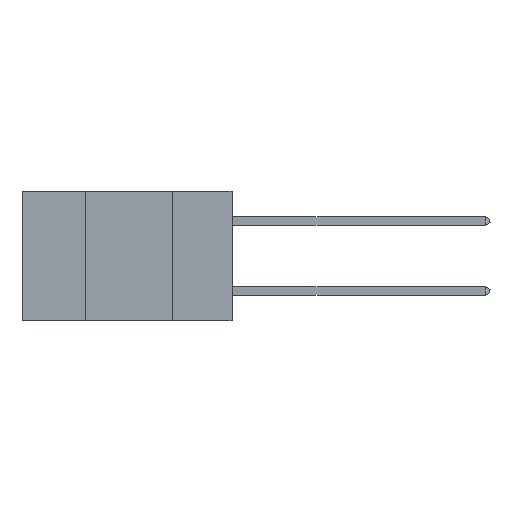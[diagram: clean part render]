
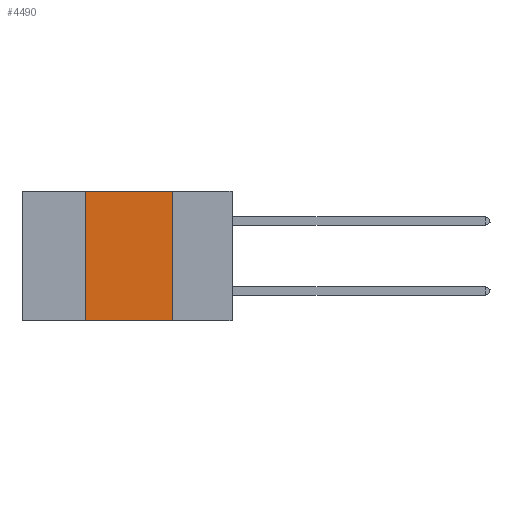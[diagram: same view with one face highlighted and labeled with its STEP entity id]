
A CAD part, left-side view. The second image highlights one B-rep face of the part: STEP entity #4490.
In plain terms, the highlighted planar face has unit normal (-1, 0, 0).
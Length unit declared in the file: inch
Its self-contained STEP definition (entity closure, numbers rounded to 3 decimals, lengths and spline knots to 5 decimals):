
#148 = PLANE ( 'NONE',  #22078 ) ;
#968 = EDGE_CURVE ( 'NONE', #27997, #3511, #27365, .T. ) ;
#1238 = CARTESIAN_POINT ( 'NONE',  ( 0., 0.17, 0. ) ) ;
#1795 = CARTESIAN_POINT ( 'NONE',  ( 0., 0.42, 0. ) ) ;
#2492 = EDGE_CURVE ( 'NONE', #27997, #30050, #5130, .T. ) ;
#2885 = ORIENTED_EDGE ( 'NONE', *, *, #16383, .F. ) ;
#3511 = VERTEX_POINT ( 'NONE', #7386 ) ;
#3553 = VECTOR ( 'NONE', #8296, 39.37008 ) ;
#4490 = ADVANCED_FACE ( 'NONE', ( #25367 ), #148, .F. ) ;
#5130 = LINE ( 'NONE', #18035, #3553 ) ;
#5459 = LINE ( 'NONE', #10058, #13651 ) ;
#6188 = CARTESIAN_POINT ( 'NONE',  ( 0., 0.17, 0. ) ) ;
#7386 = CARTESIAN_POINT ( 'NONE',  ( 0., 0.17, -0.37 ) ) ;
#8296 = DIRECTION ( 'NONE',  ( 0., 0., 1. ) ) ;
#8498 = VERTEX_POINT ( 'NONE', #1238 ) ;
#10058 = CARTESIAN_POINT ( 'NONE',  ( 0., 0.6, 0. ) ) ;
#12219 = CARTESIAN_POINT ( 'NONE',  ( 0., 0.6, 0. ) ) ;
#13433 = LINE ( 'NONE', #6188, #14620 ) ;
#13651 = VECTOR ( 'NONE', #30189, 39.37008 ) ;
#14620 = VECTOR ( 'NONE', #28639, 39.37008 ) ;
#16383 = EDGE_CURVE ( 'NONE', #8498, #3511, #13433, .T. ) ;
#18035 = CARTESIAN_POINT ( 'NONE',  ( 0., 0.42, 0. ) ) ;
#20558 = CARTESIAN_POINT ( 'NONE',  ( 0., 0.42, -0.37 ) ) ;
#21073 = EDGE_LOOP ( 'NONE', ( #2885, #28188, #26571, #30292 ) ) ;
#22078 = AXIS2_PLACEMENT_3D ( 'NONE', #12219, #29842, #29744 ) ;
#25367 = FACE_OUTER_BOUND ( 'NONE', #21073, .T. ) ;
#26350 = EDGE_CURVE ( 'NONE', #30050, #8498, #5459, .T. ) ;
#26571 = ORIENTED_EDGE ( 'NONE', *, *, #2492, .F. ) ;
#26580 = VECTOR ( 'NONE', #28399, 39.37008 ) ;
#27365 = LINE ( 'NONE', #31245, #26580 ) ;
#27997 = VERTEX_POINT ( 'NONE', #20558 ) ;
#28188 = ORIENTED_EDGE ( 'NONE', *, *, #26350, .F. ) ;
#28399 = DIRECTION ( 'NONE',  ( 0., -1., 0. ) ) ;
#28639 = DIRECTION ( 'NONE',  ( 0., 0., -1. ) ) ;
#29744 = DIRECTION ( 'NONE',  ( 0., 0., -1. ) ) ;
#29842 = DIRECTION ( 'NONE',  ( 1., 0., 0. ) ) ;
#30050 = VERTEX_POINT ( 'NONE', #1795 ) ;
#30189 = DIRECTION ( 'NONE',  ( 0., -1., 0. ) ) ;
#30292 = ORIENTED_EDGE ( 'NONE', *, *, #968, .T. ) ;
#31245 = CARTESIAN_POINT ( 'NONE',  ( 0., 0.6, -0.37 ) ) ;
